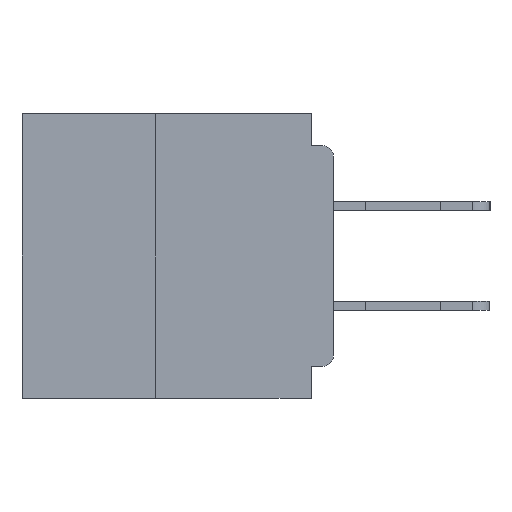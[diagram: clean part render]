
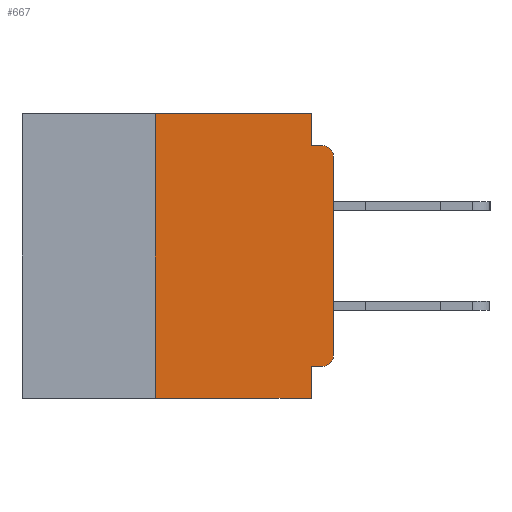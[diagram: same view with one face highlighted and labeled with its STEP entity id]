
A CAD part, left-side view. The second image highlights one B-rep face of the part: STEP entity #667.
In plain terms, the highlighted planar face has unit normal (-1, 0, 0).
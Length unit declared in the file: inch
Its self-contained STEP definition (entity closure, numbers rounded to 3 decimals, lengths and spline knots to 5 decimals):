
#543 = VERTEX_POINT ( 'NONE', #35335 ) ;
#635 = VERTEX_POINT ( 'NONE', #17761 ) ;
#667 = ADVANCED_FACE ( 'NONE', ( #23948 ), #14215, .F. ) ;
#1737 = EDGE_CURVE ( 'NONE', #635, #19277, #12894, .T. ) ;
#2042 = VERTEX_POINT ( 'NONE', #34927 ) ;
#3026 = CARTESIAN_POINT ( 'NONE',  ( 0., 0., -0.06 ) ) ;
#3051 = DIRECTION ( 'NONE',  ( 0., -1., 0. ) ) ;
#3115 = CARTESIAN_POINT ( 'NONE',  ( 0., 0., -0.34 ) ) ;
#4079 = VECTOR ( 'NONE', #26296, 39.37008 ) ;
#4186 = LINE ( 'NONE', #7023, #35399 ) ;
#4869 = DIRECTION ( 'NONE',  ( 0., -1., 0. ) ) ;
#4913 = CARTESIAN_POINT ( 'NONE',  ( 0., 0.015, -0.355 ) ) ;
#4981 = CARTESIAN_POINT ( 'NONE',  ( 0., 0., 0. ) ) ;
#5970 = VERTEX_POINT ( 'NONE', #6225 ) ;
#6225 = CARTESIAN_POINT ( 'NONE',  ( 0., 0.031, -0.045 ) ) ;
#6663 = AXIS2_PLACEMENT_3D ( 'NONE', #8551, #29818, #11586 ) ;
#7023 = CARTESIAN_POINT ( 'NONE',  ( 0., 0., -0.355 ) ) ;
#7234 = DIRECTION ( 'NONE',  ( 0., -1., 0. ) ) ;
#7881 = ORIENTED_EDGE ( 'NONE', *, *, #16907, .F. ) ;
#7990 = ORIENTED_EDGE ( 'NONE', *, *, #18306, .T. ) ;
#8551 = CARTESIAN_POINT ( 'NONE',  ( 0., 0.015, -0.06 ) ) ;
#8572 = CARTESIAN_POINT ( 'NONE',  ( 0., 0.031, 0. ) ) ;
#8639 = CARTESIAN_POINT ( 'NONE',  ( 0., 0.031, -0.4 ) ) ;
#9118 = ORIENTED_EDGE ( 'NONE', *, *, #37547, .T. ) ;
#9355 = CARTESIAN_POINT ( 'NONE',  ( 0., 0.031, -0.355 ) ) ;
#9551 = CARTESIAN_POINT ( 'NONE',  ( 0., 0.437, 0. ) ) ;
#9749 = VECTOR ( 'NONE', #4869, 39.37008 ) ;
#11586 = DIRECTION ( 'NONE',  ( 0., 0., -1. ) ) ;
#12145 = VERTEX_POINT ( 'NONE', #21160 ) ;
#12189 = VECTOR ( 'NONE', #17742, 39.37008 ) ;
#12230 = DIRECTION ( 'NONE',  ( 0., 0., -1. ) ) ;
#12590 = EDGE_CURVE ( 'NONE', #5970, #543, #26866, .T. ) ;
#12616 = DIRECTION ( 'NONE',  ( 1., 0., 0. ) ) ;
#12894 = LINE ( 'NONE', #9551, #28098 ) ;
#14139 = CARTESIAN_POINT ( 'NONE',  ( 0., 0.437, 0. ) ) ;
#14215 = PLANE ( 'NONE',  #28176 ) ;
#14449 = ORIENTED_EDGE ( 'NONE', *, *, #29174, .F. ) ;
#16907 = EDGE_CURVE ( 'NONE', #19277, #5970, #20280, .T. ) ;
#17003 = VECTOR ( 'NONE', #23218, 39.37008 ) ;
#17742 = DIRECTION ( 'NONE',  ( 0., 0., -1. ) ) ;
#17761 = CARTESIAN_POINT ( 'NONE',  ( 0., 0.25, 0. ) ) ;
#17790 = CARTESIAN_POINT ( 'NONE',  ( 0., 0.015, -0.34 ) ) ;
#18306 = EDGE_CURVE ( 'NONE', #2042, #12145, #36978, .T. ) ;
#18650 = CIRCLE ( 'NONE', #28913, 0.015 ) ;
#18856 = VECTOR ( 'NONE', #23937, 39.37008 ) ;
#18958 = VERTEX_POINT ( 'NONE', #9355 ) ;
#19277 = VERTEX_POINT ( 'NONE', #29668 ) ;
#20280 = LINE ( 'NONE', #8572, #12189 ) ;
#20847 = DIRECTION ( 'NONE',  ( 0., 0., -1. ) ) ;
#21160 = CARTESIAN_POINT ( 'NONE',  ( 0., 0.031, -0.4 ) ) ;
#21318 = ORIENTED_EDGE ( 'NONE', *, *, #26623, .T. ) ;
#22064 = ORIENTED_EDGE ( 'NONE', *, *, #12590, .F. ) ;
#23135 = CARTESIAN_POINT ( 'NONE',  ( 0., 0., -0.045 ) ) ;
#23218 = DIRECTION ( 'NONE',  ( 0., 0., 1. ) ) ;
#23937 = DIRECTION ( 'NONE',  ( 0., 0., -1. ) ) ;
#23948 = FACE_OUTER_BOUND ( 'NONE', #32812, .T. ) ;
#24624 = LINE ( 'NONE', #4981, #4079 ) ;
#26154 = VERTEX_POINT ( 'NONE', #3115 ) ;
#26296 = DIRECTION ( 'NONE',  ( 0., 0., 1. ) ) ;
#26568 = ORIENTED_EDGE ( 'NONE', *, *, #35163, .T. ) ;
#26617 = ORIENTED_EDGE ( 'NONE', *, *, #35502, .F. ) ;
#26623 = EDGE_CURVE ( 'NONE', #35071, #26154, #18650, .T. ) ;
#26866 = LINE ( 'NONE', #23135, #9749 ) ;
#27881 = LINE ( 'NONE', #8639, #18856 ) ;
#28098 = VECTOR ( 'NONE', #7234, 39.37008 ) ;
#28176 = AXIS2_PLACEMENT_3D ( 'NONE', #14139, #12616, #12230 ) ;
#28913 = AXIS2_PLACEMENT_3D ( 'NONE', #17790, #38636, #20847 ) ;
#29174 = EDGE_CURVE ( 'NONE', #2042, #635, #38906, .T. ) ;
#29668 = CARTESIAN_POINT ( 'NONE',  ( 0., 0.031, 0. ) ) ;
#29818 = DIRECTION ( 'NONE',  ( -1., 0., 0. ) ) ;
#30551 = EDGE_CURVE ( 'NONE', #18958, #12145, #27881, .T. ) ;
#32160 = ORIENTED_EDGE ( 'NONE', *, *, #30551, .F. ) ;
#32812 = EDGE_LOOP ( 'NONE', ( #9118, #26568, #22064, #7881, #34753, #14449, #7990, #32160, #26617, #21318 ) ) ;
#33609 = CIRCLE ( 'NONE', #6663, 0.015 ) ;
#33784 = VERTEX_POINT ( 'NONE', #3026 ) ;
#34753 = ORIENTED_EDGE ( 'NONE', *, *, #1737, .F. ) ;
#34927 = CARTESIAN_POINT ( 'NONE',  ( 0., 0.25, -0.4 ) ) ;
#35071 = VERTEX_POINT ( 'NONE', #4913 ) ;
#35163 = EDGE_CURVE ( 'NONE', #33784, #543, #33609, .T. ) ;
#35335 = CARTESIAN_POINT ( 'NONE',  ( 0., 0.015, -0.045 ) ) ;
#35399 = VECTOR ( 'NONE', #37179, 39.37008 ) ;
#35502 = EDGE_CURVE ( 'NONE', #35071, #18958, #4186, .T. ) ;
#36069 = VECTOR ( 'NONE', #3051, 39.37008 ) ;
#36978 = LINE ( 'NONE', #39117, #36069 ) ;
#37179 = DIRECTION ( 'NONE',  ( 0., 1., 0. ) ) ;
#37547 = EDGE_CURVE ( 'NONE', #26154, #33784, #24624, .T. ) ;
#37976 = CARTESIAN_POINT ( 'NONE',  ( 0., 0.25, -0.4 ) ) ;
#38636 = DIRECTION ( 'NONE',  ( -1., 0., 0. ) ) ;
#38906 = LINE ( 'NONE', #37976, #17003 ) ;
#39117 = CARTESIAN_POINT ( 'NONE',  ( 0., 0.437, -0.4 ) ) ;
